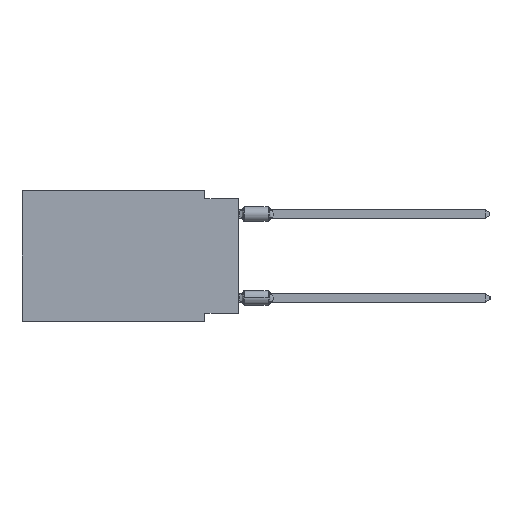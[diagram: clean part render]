
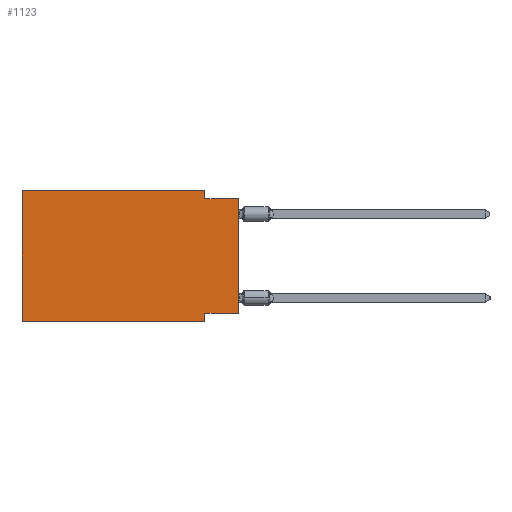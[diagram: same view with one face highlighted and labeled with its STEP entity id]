
A CAD part, left-side view. The second image highlights one B-rep face of the part: STEP entity #1123.
In plain terms, the highlighted planar face has unit normal (-1, 0, 0).
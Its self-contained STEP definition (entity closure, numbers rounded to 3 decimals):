
#21 = DIRECTION ( 'NONE',  ( 0., -1., 0. ) ) ;
#574 = VECTOR ( 'NONE', #3369, 1000. ) ;
#1123 = ADVANCED_FACE ( 'NONE', ( #10589 ), #7413, .F. ) ;
#1744 = CARTESIAN_POINT ( 'NONE',  ( 0., 2.54, 0. ) ) ;
#3080 = CARTESIAN_POINT ( 'NONE',  ( 0., 16.383, 0. ) ) ;
#3369 = DIRECTION ( 'NONE',  ( 0., 0., 1. ) ) ;
#3604 = EDGE_CURVE ( 'NONE', #14527, #10531, #18383, .T. ) ;
#3764 = DIRECTION ( 'NONE',  ( 1., 0., 0. ) ) ;
#3940 = DIRECTION ( 'NONE',  ( 0., -1., 0. ) ) ;
#4599 = CARTESIAN_POINT ( 'NONE',  ( 0., 16.383, 0. ) ) ;
#4822 = CARTESIAN_POINT ( 'NONE',  ( 0., 0., -0.635 ) ) ;
#5002 = ORIENTED_EDGE ( 'NONE', *, *, #3604, .F. ) ;
#6152 = VERTEX_POINT ( 'NONE', #11095 ) ;
#7109 = VERTEX_POINT ( 'NONE', #4822 ) ;
#7413 = PLANE ( 'NONE',  #14583 ) ;
#7521 = ORIENTED_EDGE ( 'NONE', *, *, #23838, .F. ) ;
#7907 = VECTOR ( 'NONE', #21, 1000. ) ;
#9190 = ORIENTED_EDGE ( 'NONE', *, *, #18519, .F. ) ;
#9273 = CARTESIAN_POINT ( 'NONE',  ( 0., 2.54, -9.906 ) ) ;
#9500 = LINE ( 'NONE', #9273, #17056 ) ;
#9520 = EDGE_CURVE ( 'NONE', #35112, #7109, #30187, .T. ) ;
#9970 = VECTOR ( 'NONE', #33986, 1000. ) ;
#10034 = ORIENTED_EDGE ( 'NONE', *, *, #34629, .F. ) ;
#10531 = VERTEX_POINT ( 'NONE', #1744 ) ;
#10589 = FACE_OUTER_BOUND ( 'NONE', #15120, .T. ) ;
#11095 = CARTESIAN_POINT ( 'NONE',  ( 0., 2.54, -9.906 ) ) ;
#11247 = EDGE_CURVE ( 'NONE', #31769, #7109, #11398, .T. ) ;
#11398 = LINE ( 'NONE', #22543, #574 ) ;
#13890 = CARTESIAN_POINT ( 'NONE',  ( 0., 2.54, 0. ) ) ;
#14527 = VERTEX_POINT ( 'NONE', #24779 ) ;
#14583 = AXIS2_PLACEMENT_3D ( 'NONE', #22226, #3764, #18584 ) ;
#15120 = EDGE_LOOP ( 'NONE', ( #25559, #43421, #34757, #5002, #10034, #31781, #9190, #7521 ) ) ;
#16563 = DIRECTION ( 'NONE',  ( 0., 0., -1. ) ) ;
#17056 = VECTOR ( 'NONE', #16563, 1000. ) ;
#18244 = LINE ( 'NONE', #13890, #38952 ) ;
#18383 = LINE ( 'NONE', #3080, #22905 ) ;
#18519 = EDGE_CURVE ( 'NONE', #23304, #6152, #9500, .T. ) ;
#18584 = DIRECTION ( 'NONE',  ( 0., 0., -1. ) ) ;
#19171 = LINE ( 'NONE', #4599, #9970 ) ;
#21044 = LINE ( 'NONE', #43148, #27240 ) ;
#22180 = VECTOR ( 'NONE', #3940, 1000. ) ;
#22226 = CARTESIAN_POINT ( 'NONE',  ( 0., 16.383, 0. ) ) ;
#22543 = CARTESIAN_POINT ( 'NONE',  ( 0., 0., 0. ) ) ;
#22905 = VECTOR ( 'NONE', #44353, 1000. ) ;
#23304 = VERTEX_POINT ( 'NONE', #23556 ) ;
#23556 = CARTESIAN_POINT ( 'NONE',  ( 0., 2.54, -9.271 ) ) ;
#23838 = EDGE_CURVE ( 'NONE', #31769, #23304, #21044, .T. ) ;
#24779 = CARTESIAN_POINT ( 'NONE',  ( 0., 16.383, 0. ) ) ;
#25559 = ORIENTED_EDGE ( 'NONE', *, *, #11247, .T. ) ;
#26012 = CARTESIAN_POINT ( 'NONE',  ( 0., 16.383, -9.906 ) ) ;
#26550 = CARTESIAN_POINT ( 'NONE',  ( 0., 16.383, -9.906 ) ) ;
#27240 = VECTOR ( 'NONE', #43386, 1000. ) ;
#30187 = LINE ( 'NONE', #44978, #22180 ) ;
#30320 = DIRECTION ( 'NONE',  ( 0., 0., -1. ) ) ;
#31769 = VERTEX_POINT ( 'NONE', #35387 ) ;
#31781 = ORIENTED_EDGE ( 'NONE', *, *, #40967, .T. ) ;
#33986 = DIRECTION ( 'NONE',  ( 0., 0., 1. ) ) ;
#34629 = EDGE_CURVE ( 'NONE', #47337, #14527, #19171, .T. ) ;
#34757 = ORIENTED_EDGE ( 'NONE', *, *, #41350, .F. ) ;
#35112 = VERTEX_POINT ( 'NONE', #38989 ) ;
#35387 = CARTESIAN_POINT ( 'NONE',  ( 0., 0., -9.271 ) ) ;
#38952 = VECTOR ( 'NONE', #30320, 1000. ) ;
#38989 = CARTESIAN_POINT ( 'NONE',  ( 0., 2.54, -0.635 ) ) ;
#40967 = EDGE_CURVE ( 'NONE', #47337, #6152, #45418, .T. ) ;
#41350 = EDGE_CURVE ( 'NONE', #10531, #35112, #18244, .T. ) ;
#43148 = CARTESIAN_POINT ( 'NONE',  ( 0., 0., -9.271 ) ) ;
#43386 = DIRECTION ( 'NONE',  ( 0., 1., 0. ) ) ;
#43421 = ORIENTED_EDGE ( 'NONE', *, *, #9520, .F. ) ;
#44353 = DIRECTION ( 'NONE',  ( 0., -1., 0. ) ) ;
#44978 = CARTESIAN_POINT ( 'NONE',  ( 0., 0., -0.635 ) ) ;
#45418 = LINE ( 'NONE', #26012, #7907 ) ;
#47337 = VERTEX_POINT ( 'NONE', #26550 ) ;
